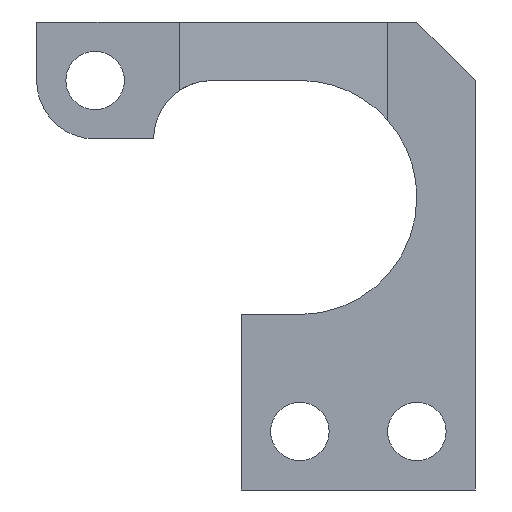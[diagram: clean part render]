
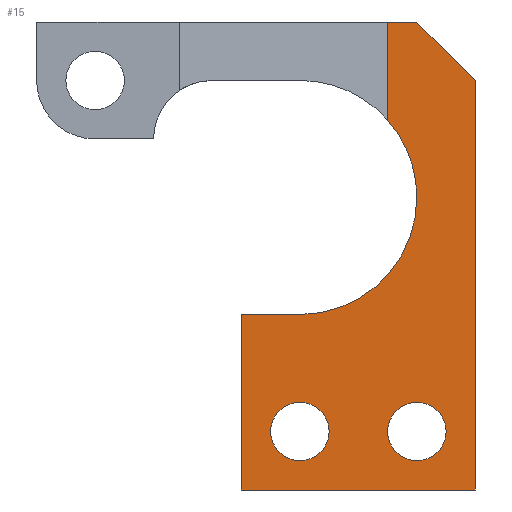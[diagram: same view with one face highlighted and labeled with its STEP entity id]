
A CAD part, left-side view. The second image highlights one B-rep face of the part: STEP entity #15.
In plain terms, the highlighted planar face has unit normal (-1, 0, 0).
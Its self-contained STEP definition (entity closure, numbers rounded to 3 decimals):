
#1 = ORIENTED_EDGE ( 'NONE', *, *, #258, .F. ) ;
#15 = ADVANCED_FACE ( 'NONE', ( #855, #843, #853 ), #724, .T. ) ;
#26 = AXIS2_PLACEMENT_3D ( 'NONE', #134, #132, #129 ) ;
#31 = EDGE_CURVE ( 'NONE', #1204, #1155, #842, .T. ) ;
#36 = AXIS2_PLACEMENT_3D ( 'NONE', #209, #1197, #181 ) ;
#64 = CARTESIAN_POINT ( 'NONE',  ( 1.875, -7.175, 4.25 ) ) ;
#66 = DIRECTION ( 'NONE',  ( 0., 0., -1. ) ) ;
#80 = CARTESIAN_POINT ( 'NONE',  ( 1.875, 4.075, -4.654 ) ) ;
#81 = CARTESIAN_POINT ( 'NONE',  ( 1.875, -0.058, 4.25 ) ) ;
#83 = DIRECTION ( 'NONE',  ( 0., 0.707, 0.707 ) ) ;
#97 = CARTESIAN_POINT ( 'NONE',  ( 1.875, -18.425, -15.904 ) ) ;
#112 = DIRECTION ( 'NONE',  ( 0., 0., -1. ) ) ;
#115 = ORIENTED_EDGE ( 'NONE', *, *, #205, .T. ) ;
#117 = ORIENTED_EDGE ( 'NONE', *, *, #271, .F. ) ;
#129 = DIRECTION ( 'NONE',  ( 0., 0., 1. ) ) ;
#132 = DIRECTION ( 'NONE',  ( -1., 0., 0. ) ) ;
#134 = CARTESIAN_POINT ( 'NONE',  ( 1.875, -10.925, -8.404 ) ) ;
#139 = CARTESIAN_POINT ( 'NONE',  ( 1.875, -18.425, -15.904 ) ) ;
#141 = ORIENTED_EDGE ( 'NONE', *, *, #658, .F. ) ;
#144 = VERTEX_POINT ( 'NONE', #394 ) ;
#145 = CARTESIAN_POINT ( 'NONE',  ( 1.875, 4.075, -12.154 ) ) ;
#148 = CARTESIAN_POINT ( 'NONE',  ( 1.875, -25.414, 29.606 ) ) ;
#151 = VERTEX_POINT ( 'NONE', #313 ) ;
#153 = AXIS2_PLACEMENT_3D ( 'NONE', #81, #694, #914 ) ;
#176 = CARTESIAN_POINT ( 'NONE',  ( 1.875, 4.075, 6.596 ) ) ;
#177 = EDGE_CURVE ( 'NONE', #917, #882, #780, .T. ) ;
#181 = DIRECTION ( 'NONE',  ( 0., 0., 1. ) ) ;
#186 = CARTESIAN_POINT ( 'NONE',  ( 1.875, -7.175, 44.096 ) ) ;
#190 = ORIENTED_EDGE ( 'NONE', *, *, #247, .T. ) ;
#196 = EDGE_CURVE ( 'NONE', #144, #151, #771, .T. ) ;
#197 = EDGE_CURVE ( 'NONE', #340, #1003, #798, .T. ) ;
#205 = EDGE_CURVE ( 'NONE', #340, #1204, #765, .T. ) ;
#209 = CARTESIAN_POINT ( 'NONE',  ( 1.875, 4.075, -8.404 ) ) ;
#214 = EDGE_CURVE ( 'NONE', #1155, #1089, #752, .T. ) ;
#215 = ORIENTED_EDGE ( 'NONE', *, *, #244, .T. ) ;
#244 = EDGE_CURVE ( 'NONE', #1089, #1125, #722, .T. ) ;
#247 = EDGE_CURVE ( 'NONE', #1125, #1142, #744, .T. ) ;
#258 = EDGE_CURVE ( 'NONE', #487, #1142, #706, .T. ) ;
#271 = EDGE_CURVE ( 'NONE', #1085, #487, #703, .T. ) ;
#274 = EDGE_CURVE ( 'NONE', #1003, #1085, #707, .T. ) ;
#313 = CARTESIAN_POINT ( 'NONE',  ( 1.875, -10.925, -12.154 ) ) ;
#339 = AXIS2_PLACEMENT_3D ( 'NONE', #1194, #1191, #1181 ) ;
#340 = VERTEX_POINT ( 'NONE', #1053 ) ;
#352 = AXIS2_PLACEMENT_3D ( 'NONE', #1176, #1172, #1171 ) ;
#394 = CARTESIAN_POINT ( 'NONE',  ( 1.875, -10.925, -4.654 ) ) ;
#411 = EDGE_CURVE ( 'NONE', #882, #917, #629, .T. ) ;
#456 = CARTESIAN_POINT ( 'NONE',  ( 1.875, -10.925, 44.096 ) ) ;
#457 = DIRECTION ( 'NONE',  ( 0., 0., 1. ) ) ;
#465 = DIRECTION ( 'NONE',  ( -1., 0., 0. ) ) ;
#471 = CARTESIAN_POINT ( 'NONE',  ( 1.875, -10.925, -8.404 ) ) ;
#480 = CIRCLE ( 'NONE', #675, 3.75 ) ;
#487 = VERTEX_POINT ( 'NONE', #813 ) ;
#512 = ORIENTED_EDGE ( 'NONE', *, *, #177, .F. ) ;
#584 = ORIENTED_EDGE ( 'NONE', *, *, #411, .F. ) ;
#605 = CARTESIAN_POINT ( 'NONE',  ( 1.875, -7.175, 31.518 ) ) ;
#629 = CIRCLE ( 'NONE', #833, 3.75 ) ;
#658 = EDGE_CURVE ( 'NONE', #151, #144, #480, .T. ) ;
#675 = AXIS2_PLACEMENT_3D ( 'NONE', #471, #465, #457 ) ;
#690 = VECTOR ( 'NONE', #1162, 1000. ) ;
#694 = DIRECTION ( 'NONE',  ( -1., 0., 0. ) ) ;
#703 = LINE ( 'NONE', #1146, #713 ) ;
#705 = VECTOR ( 'NONE', #1164, 1000. ) ;
#706 = LINE ( 'NONE', #1202, #705 ) ;
#707 = LINE ( 'NONE', #1160, #690 ) ;
#708 = CARTESIAN_POINT ( 'NONE',  ( 1.875, -10.925, 21.596 ) ) ;
#713 = VECTOR ( 'NONE', #1145, 1000. ) ;
#722 = CIRCLE ( 'NONE', #339, 15. ) ;
#724 = PLANE ( 'NONE',  #153 ) ;
#733 = VECTOR ( 'NONE', #66, 1000. ) ;
#744 = CIRCLE ( 'NONE', #352, 15. ) ;
#750 = VECTOR ( 'NONE', #83, 1000. ) ;
#752 = LINE ( 'NONE', #64, #733 ) ;
#756 = VECTOR ( 'NONE', #112, 1000. ) ;
#761 = DIRECTION ( 'NONE',  ( 0., 1., 0. ) ) ;
#765 = LINE ( 'NONE', #148, #750 ) ;
#771 = CIRCLE ( 'NONE', #26, 3.75 ) ;
#776 = ORIENTED_EDGE ( 'NONE', *, *, #214, .T. ) ;
#780 = CIRCLE ( 'NONE', #36, 3.75 ) ;
#792 = ORIENTED_EDGE ( 'NONE', *, *, #274, .F. ) ;
#798 = LINE ( 'NONE', #139, #756 ) ;
#801 = CARTESIAN_POINT ( 'NONE',  ( 1.875, -18.425, 44.096 ) ) ;
#813 = CARTESIAN_POINT ( 'NONE',  ( 1.875, 11.575, 6.596 ) ) ;
#827 = ORIENTED_EDGE ( 'NONE', *, *, #31, .T. ) ;
#833 = AXIS2_PLACEMENT_3D ( 'NONE', #932, #929, #920 ) ;
#842 = LINE ( 'NONE', #801, #848 ) ;
#843 = FACE_BOUND ( 'NONE', #944, .T. ) ;
#848 = VECTOR ( 'NONE', #761, 1000. ) ;
#853 = FACE_OUTER_BOUND ( 'NONE', #1074, .T. ) ;
#855 = FACE_BOUND ( 'NONE', #924, .T. ) ;
#882 = VERTEX_POINT ( 'NONE', #145 ) ;
#914 = DIRECTION ( 'NONE',  ( 0., 0., 1. ) ) ;
#917 = VERTEX_POINT ( 'NONE', #80 ) ;
#920 = DIRECTION ( 'NONE',  ( 0., 0., 1. ) ) ;
#924 = EDGE_LOOP ( 'NONE', ( #512, #584 ) ) ;
#929 = DIRECTION ( 'NONE',  ( -1., 0., 0. ) ) ;
#932 = CARTESIAN_POINT ( 'NONE',  ( 1.875, 4.075, -8.404 ) ) ;
#944 = EDGE_LOOP ( 'NONE', ( #949, #141 ) ) ;
#949 = ORIENTED_EDGE ( 'NONE', *, *, #196, .F. ) ;
#999 = CARTESIAN_POINT ( 'NONE',  ( 1.875, 11.575, -15.904 ) ) ;
#1003 = VERTEX_POINT ( 'NONE', #97 ) ;
#1053 = CARTESIAN_POINT ( 'NONE',  ( 1.875, -18.425, 36.596 ) ) ;
#1074 = EDGE_LOOP ( 'NONE', ( #1169, #115, #827, #776, #215, #190, #1, #117, #792 ) ) ;
#1085 = VERTEX_POINT ( 'NONE', #999 ) ;
#1089 = VERTEX_POINT ( 'NONE', #605 ) ;
#1125 = VERTEX_POINT ( 'NONE', #708 ) ;
#1142 = VERTEX_POINT ( 'NONE', #176 ) ;
#1145 = DIRECTION ( 'NONE',  ( 0., 0., 1. ) ) ;
#1146 = CARTESIAN_POINT ( 'NONE',  ( 1.875, 11.575, -15.904 ) ) ;
#1155 = VERTEX_POINT ( 'NONE', #186 ) ;
#1160 = CARTESIAN_POINT ( 'NONE',  ( 1.875, 11.575, -15.904 ) ) ;
#1162 = DIRECTION ( 'NONE',  ( 0., 1., 0. ) ) ;
#1164 = DIRECTION ( 'NONE',  ( 0., -1., 0. ) ) ;
#1169 = ORIENTED_EDGE ( 'NONE', *, *, #197, .F. ) ;
#1171 = DIRECTION ( 'NONE',  ( 0., 0., 1. ) ) ;
#1172 = DIRECTION ( 'NONE',  ( 1., 0., 0. ) ) ;
#1176 = CARTESIAN_POINT ( 'NONE',  ( 1.875, 4.075, 21.596 ) ) ;
#1181 = DIRECTION ( 'NONE',  ( 0., 0., 1. ) ) ;
#1191 = DIRECTION ( 'NONE',  ( 1., 0., 0. ) ) ;
#1194 = CARTESIAN_POINT ( 'NONE',  ( 1.875, 4.075, 21.596 ) ) ;
#1197 = DIRECTION ( 'NONE',  ( -1., 0., 0. ) ) ;
#1202 = CARTESIAN_POINT ( 'NONE',  ( 1.875, 11.575, 6.596 ) ) ;
#1204 = VERTEX_POINT ( 'NONE', #456 ) ;
